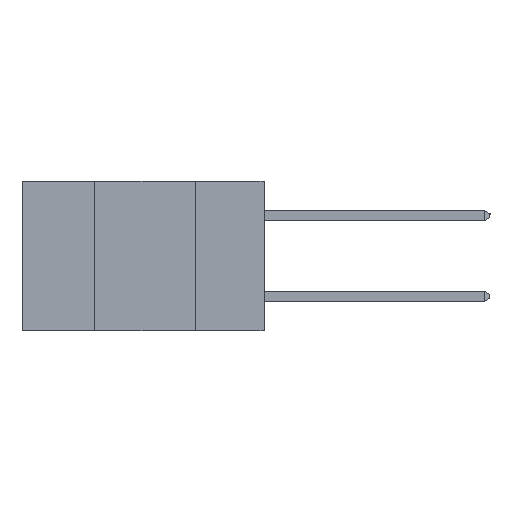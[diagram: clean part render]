
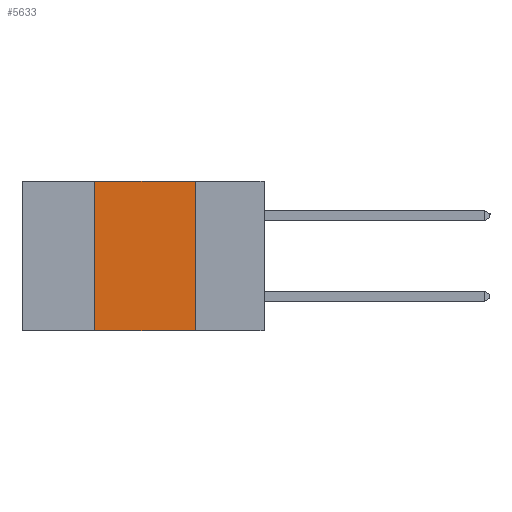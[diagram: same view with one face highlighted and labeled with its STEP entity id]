
A CAD part, left-side view. The second image highlights one B-rep face of the part: STEP entity #5633.
In plain terms, the highlighted planar face has unit normal (-1, 0, 0).
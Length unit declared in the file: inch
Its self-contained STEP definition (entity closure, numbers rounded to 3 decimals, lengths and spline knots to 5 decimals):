
#149 = DIRECTION ( 'NONE',  ( 0., 0., -1. ) ) ;
#422 = DIRECTION ( 'NONE',  ( 1., 0., 0. ) ) ;
#488 = FACE_OUTER_BOUND ( 'NONE', #12032, .T. ) ;
#967 = EDGE_CURVE ( 'NONE', #1286, #10900, #8095, .T. ) ;
#972 = LINE ( 'NONE', #4725, #2056 ) ;
#1286 = VERTEX_POINT ( 'NONE', #11539 ) ;
#1288 = AXIS2_PLACEMENT_3D ( 'NONE', #9590, #422, #3518 ) ;
#1997 = CARTESIAN_POINT ( 'NONE',  ( 0., 0.42, -0.37 ) ) ;
#2056 = VECTOR ( 'NONE', #3813, 39.37008 ) ;
#2480 = CARTESIAN_POINT ( 'NONE',  ( 0., 0.6, -0.37 ) ) ;
#2667 = PLANE ( 'NONE',  #1288 ) ;
#2880 = VERTEX_POINT ( 'NONE', #10902 ) ;
#3056 = ORIENTED_EDGE ( 'NONE', *, *, #12065, .F. ) ;
#3113 = CARTESIAN_POINT ( 'NONE',  ( 0., 0.6, 0. ) ) ;
#3518 = DIRECTION ( 'NONE',  ( 0., 0., -1. ) ) ;
#3775 = EDGE_CURVE ( 'NONE', #10580, #1286, #972, .T. ) ;
#3813 = DIRECTION ( 'NONE',  ( 0., 0., 1. ) ) ;
#4140 = CARTESIAN_POINT ( 'NONE',  ( 0., 0.17, 0. ) ) ;
#4400 = ORIENTED_EDGE ( 'NONE', *, *, #11643, .T. ) ;
#4725 = CARTESIAN_POINT ( 'NONE',  ( 0., 0.42, -0.37 ) ) ;
#5140 = VECTOR ( 'NONE', #6605, 39.37008 ) ;
#5218 = LINE ( 'NONE', #12189, #12857 ) ;
#5350 = VECTOR ( 'NONE', #8943, 39.37008 ) ;
#5633 = ADVANCED_FACE ( 'NONE', ( #488 ), #2667, .F. ) ;
#5841 = ORIENTED_EDGE ( 'NONE', *, *, #3775, .F. ) ;
#6605 = DIRECTION ( 'NONE',  ( 0., -1., 0. ) ) ;
#8095 = LINE ( 'NONE', #3113, #5350 ) ;
#8346 = ORIENTED_EDGE ( 'NONE', *, *, #967, .F. ) ;
#8943 = DIRECTION ( 'NONE',  ( 0., -1., 0. ) ) ;
#9590 = CARTESIAN_POINT ( 'NONE',  ( 0., 0.6, 0. ) ) ;
#9597 = LINE ( 'NONE', #2480, #5140 ) ;
#10580 = VERTEX_POINT ( 'NONE', #1997 ) ;
#10900 = VERTEX_POINT ( 'NONE', #4140 ) ;
#10902 = CARTESIAN_POINT ( 'NONE',  ( 0., 0.17, -0.37 ) ) ;
#11539 = CARTESIAN_POINT ( 'NONE',  ( 0., 0.42, 0. ) ) ;
#11643 = EDGE_CURVE ( 'NONE', #10580, #2880, #9597, .T. ) ;
#12032 = EDGE_LOOP ( 'NONE', ( #3056, #8346, #5841, #4400 ) ) ;
#12065 = EDGE_CURVE ( 'NONE', #10900, #2880, #5218, .T. ) ;
#12189 = CARTESIAN_POINT ( 'NONE',  ( 0., 0.17, -0.37 ) ) ;
#12857 = VECTOR ( 'NONE', #149, 39.37008 ) ;
